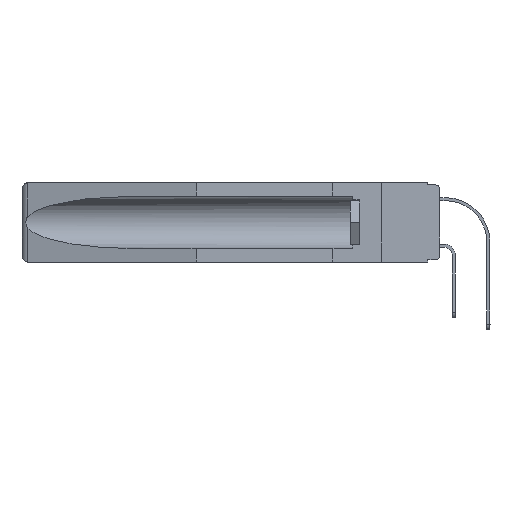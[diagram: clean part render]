
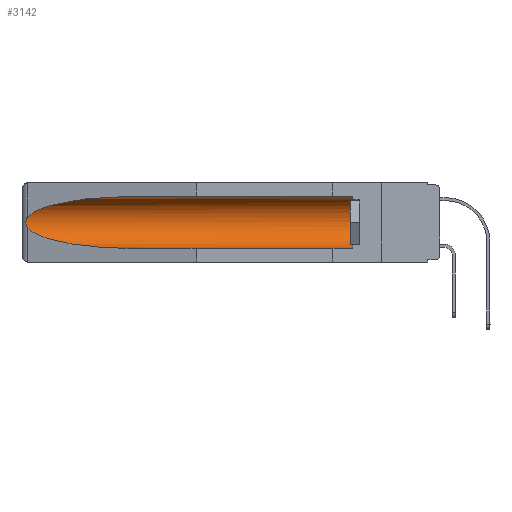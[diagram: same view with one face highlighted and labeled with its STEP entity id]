
A CAD part, left-side view. The second image highlights one B-rep face of the part: STEP entity #3142.
In plain terms, the highlighted cylindrical face has radius 2.857 mm (diameter 5.715 mm), a partial arc.
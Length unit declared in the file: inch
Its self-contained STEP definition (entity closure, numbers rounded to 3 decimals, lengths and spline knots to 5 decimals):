
#122 = CARTESIAN_POINT ( 'NONE',  ( 0.26655, 1.53094, -0.18657 ) ) ;
#988 = CARTESIAN_POINT ( 'NONE',  ( 0.26537, 1.52718, -0.19328 ) ) ;
#1451 = CARTESIAN_POINT ( 'NONE',  ( 0.155, -0.30754, -0.284 ) ) ;
#1660 = B_SPLINE_CURVE_WITH_KNOTS ( 'NONE', 3,
 ( #15585, #1700, #8885, #15467, #15694, #19048, #17257, #122, #5213, #1912 ),
 .UNSPECIFIED., .F., .F.,
 ( 4, 2, 2, 2, 4 ),
 ( 0., 0.00029, 0.00058, 0.00087, 0.00117 ),
 .UNSPECIFIED. ) ;
#1700 = CARTESIAN_POINT ( 'NONE',  ( 0.26597, 1.52961, -0.15275 ) ) ;
#1912 = CARTESIAN_POINT ( 'NONE',  ( 0.26537, 1.52718, -0.19328 ) ) ;
#2344 = DIRECTION ( 'NONE',  ( 0., 0., 1. ) ) ;
#2969 = VERTEX_POINT ( 'NONE', #16905 ) ;
#3142 = ADVANCED_FACE ( 'NONE', ( #3726 ), #4052, .F. ) ;
#3218 =( BOUNDED_CURVE ( )  B_SPLINE_CURVE ( 3, ( #17493, #17592, #12535, #12436 ),
 .UNSPECIFIED., .F., .T. ) 
 B_SPLINE_CURVE_WITH_KNOTS ( ( 4, 4 ),
 ( 4.71239, 6.08839 ),
 .UNSPECIFIED. ) 
 CURVE ( )  GEOMETRIC_REPRESENTATION_ITEM ( )  RATIONAL_B_SPLINE_CURVE ( ( 1., 0.848, 0.848, 1. ) ) 
 REPRESENTATION_ITEM ( '' )  );
#3228 = VERTEX_POINT ( 'NONE', #988 ) ;
#3240 = CARTESIAN_POINT ( 'NONE',  ( 0.155, -0.30754, -0.059 ) ) ;
#3686 = CARTESIAN_POINT ( 'NONE',  ( 0.26537, 1.52718, -0.14972 ) ) ;
#3726 = FACE_OUTER_BOUND ( 'NONE', #18251, .T. ) ;
#4052 = CYLINDRICAL_SURFACE ( 'NONE', #12679, 0.1125 ) ;
#5213 = CARTESIAN_POINT ( 'NONE',  ( 0.26597, 1.5296, -0.19026 ) ) ;
#5537 = CIRCLE ( 'NONE', #9089, 0.1125 ) ;
#5662 = ORIENTED_EDGE ( 'NONE', *, *, #10093, .T. ) ;
#6104 =( BOUNDED_CURVE ( )  B_SPLINE_CURVE ( 3, ( #18939, #12206, #15475, #19057 ),
 .UNSPECIFIED., .F., .T. ) 
 B_SPLINE_CURVE_WITH_KNOTS ( ( 4, 4 ),
 ( 0.1948, 1.5708 ),
 .UNSPECIFIED. ) 
 CURVE ( )  GEOMETRIC_REPRESENTATION_ITEM ( )  RATIONAL_B_SPLINE_CURVE ( ( 1., 0.848, 0.848, 1. ) ) 
 REPRESENTATION_ITEM ( '' )  );
#6524 = EDGE_CURVE ( 'NONE', #18965, #19466, #9721, .T. ) ;
#6853 = VERTEX_POINT ( 'NONE', #19526 ) ;
#6949 = ORIENTED_EDGE ( 'NONE', *, *, #17644, .T. ) ;
#8309 = CARTESIAN_POINT ( 'NONE',  ( 0.155, 0.126, -0.1715 ) ) ;
#8885 = CARTESIAN_POINT ( 'NONE',  ( 0.26654, 1.53092, -0.15636 ) ) ;
#9089 = AXIS2_PLACEMENT_3D ( 'NONE', #8309, #18497, #16805 ) ;
#9304 = ORIENTED_EDGE ( 'NONE', *, *, #6524, .T. ) ;
#9721 = LINE ( 'NONE', #3240, #10510 ) ;
#10093 = EDGE_CURVE ( 'NONE', #3228, #2969, #6104, .T. ) ;
#10439 = EDGE_CURVE ( 'NONE', #6853, #2969, #11533, .T. ) ;
#10510 = VECTOR ( 'NONE', #11496, 39.37008 ) ;
#10533 = CARTESIAN_POINT ( 'NONE',  ( 0.155, -0.30754, -0.1715 ) ) ;
#11496 = DIRECTION ( 'NONE',  ( 0., 1., 0. ) ) ;
#11533 = LINE ( 'NONE', #1451, #14882 ) ;
#12206 = CARTESIAN_POINT ( 'NONE',  ( 0.25451, 1.48313, -0.24835 ) ) ;
#12436 = CARTESIAN_POINT ( 'NONE',  ( 0.26537, 1.52718, -0.14972 ) ) ;
#12535 = CARTESIAN_POINT ( 'NONE',  ( 0.25451, 1.48313, -0.09465 ) ) ;
#12679 = AXIS2_PLACEMENT_3D ( 'NONE', #10533, #15782, #2344 ) ;
#13151 = CARTESIAN_POINT ( 'NONE',  ( 0.155, 0.126, -0.059 ) ) ;
#13221 = EDGE_CURVE ( 'NONE', #6853, #18965, #5537, .T. ) ;
#13295 = ORIENTED_EDGE ( 'NONE', *, *, #19709, .T. ) ;
#13302 = ORIENTED_EDGE ( 'NONE', *, *, #13221, .T. ) ;
#14882 = VECTOR ( 'NONE', #18381, 39.37008 ) ;
#14981 = ORIENTED_EDGE ( 'NONE', *, *, #10439, .F. ) ;
#15467 = CARTESIAN_POINT ( 'NONE',  ( 0.2673, 1.5327, -0.16383 ) ) ;
#15475 = CARTESIAN_POINT ( 'NONE',  ( 0.21114, 1.30732, -0.284 ) ) ;
#15585 = CARTESIAN_POINT ( 'NONE',  ( 0.26537, 1.52718, -0.14972 ) ) ;
#15694 = CARTESIAN_POINT ( 'NONE',  ( 0.2675, 1.53308, -0.16763 ) ) ;
#15782 = DIRECTION ( 'NONE',  ( 0., 1., 0. ) ) ;
#16803 = VERTEX_POINT ( 'NONE', #3686 ) ;
#16805 = DIRECTION ( 'NONE',  ( 0., 0., 1. ) ) ;
#16905 = CARTESIAN_POINT ( 'NONE',  ( 0.155, 1.07973, -0.284 ) ) ;
#17257 = CARTESIAN_POINT ( 'NONE',  ( 0.2673, 1.53269, -0.17917 ) ) ;
#17493 = CARTESIAN_POINT ( 'NONE',  ( 0.155, 1.07973, -0.059 ) ) ;
#17592 = CARTESIAN_POINT ( 'NONE',  ( 0.21114, 1.30732, -0.059 ) ) ;
#17644 = EDGE_CURVE ( 'NONE', #16803, #3228, #1660, .T. ) ;
#18251 = EDGE_LOOP ( 'NONE', ( #13295, #6949, #5662, #14981, #13302, #9304 ) ) ;
#18381 = DIRECTION ( 'NONE',  ( 0., 1., 0. ) ) ;
#18497 = DIRECTION ( 'NONE',  ( 0., -1., 0. ) ) ;
#18939 = CARTESIAN_POINT ( 'NONE',  ( 0.26537, 1.52718, -0.19328 ) ) ;
#18965 = VERTEX_POINT ( 'NONE', #13151 ) ;
#19048 = CARTESIAN_POINT ( 'NONE',  ( 0.2675, 1.53308, -0.17534 ) ) ;
#19057 = CARTESIAN_POINT ( 'NONE',  ( 0.155, 1.07973, -0.284 ) ) ;
#19466 = VERTEX_POINT ( 'NONE', #19858 ) ;
#19526 = CARTESIAN_POINT ( 'NONE',  ( 0.155, 0.126, -0.284 ) ) ;
#19709 = EDGE_CURVE ( 'NONE', #19466, #16803, #3218, .T. ) ;
#19858 = CARTESIAN_POINT ( 'NONE',  ( 0.155, 1.07973, -0.059 ) ) ;
